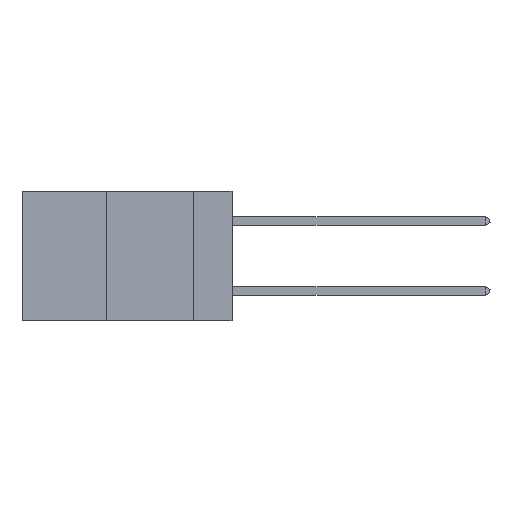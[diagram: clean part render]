
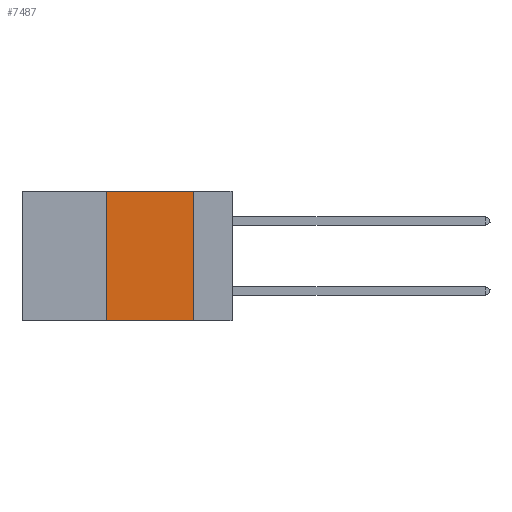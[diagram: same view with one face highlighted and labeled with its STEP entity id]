
A CAD part, left-side view. The second image highlights one B-rep face of the part: STEP entity #7487.
In plain terms, the highlighted planar face has unit normal (-1, 0, 0).
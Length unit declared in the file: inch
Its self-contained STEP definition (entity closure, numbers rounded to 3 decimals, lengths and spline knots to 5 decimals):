
#118 = VECTOR ( 'NONE', #20390, 39.37008 ) ;
#226 = ORIENTED_EDGE ( 'NONE', *, *, #33072, .F. ) ;
#620 = PLANE ( 'NONE',  #11487 ) ;
#1756 = LINE ( 'NONE', #30746, #118 ) ;
#3171 = VECTOR ( 'NONE', #6409, 39.37008 ) ;
#4182 = EDGE_CURVE ( 'NONE', #19419, #30702, #10071, .T. ) ;
#4533 = CARTESIAN_POINT ( 'NONE',  ( 0., 0.11, 0. ) ) ;
#4989 = CARTESIAN_POINT ( 'NONE',  ( 0., 0.6, -0.37 ) ) ;
#5253 = LINE ( 'NONE', #30614, #9282 ) ;
#5281 = CARTESIAN_POINT ( 'NONE',  ( 0., 0.36, -0.37 ) ) ;
#6409 = DIRECTION ( 'NONE',  ( 0., 0., 1. ) ) ;
#6517 = LINE ( 'NONE', #4989, #19477 ) ;
#6552 = CARTESIAN_POINT ( 'NONE',  ( 0., 0.11, -0.37 ) ) ;
#7487 = ADVANCED_FACE ( 'NONE', ( #15484 ), #620, .F. ) ;
#8469 = EDGE_CURVE ( 'NONE', #19419, #27528, #6517, .T. ) ;
#9282 = VECTOR ( 'NONE', #9524, 39.37008 ) ;
#9524 = DIRECTION ( 'NONE',  ( 0., 0., -1. ) ) ;
#9711 = VERTEX_POINT ( 'NONE', #4533 ) ;
#10071 = LINE ( 'NONE', #16402, #3171 ) ;
#11487 = AXIS2_PLACEMENT_3D ( 'NONE', #21248, #29193, #29083 ) ;
#11657 = CARTESIAN_POINT ( 'NONE',  ( 0., 0.36, 0. ) ) ;
#13347 = ORIENTED_EDGE ( 'NONE', *, *, #4182, .F. ) ;
#15484 = FACE_OUTER_BOUND ( 'NONE', #20965, .T. ) ;
#16402 = CARTESIAN_POINT ( 'NONE',  ( 0., 0.36, 0. ) ) ;
#18621 = EDGE_CURVE ( 'NONE', #9711, #27528, #5253, .T. ) ;
#19419 = VERTEX_POINT ( 'NONE', #5281 ) ;
#19477 = VECTOR ( 'NONE', #23463, 39.37008 ) ;
#20125 = ORIENTED_EDGE ( 'NONE', *, *, #18621, .F. ) ;
#20390 = DIRECTION ( 'NONE',  ( 0., -1., 0. ) ) ;
#20965 = EDGE_LOOP ( 'NONE', ( #20125, #226, #13347, #32925 ) ) ;
#21248 = CARTESIAN_POINT ( 'NONE',  ( 0., 0.6, 0. ) ) ;
#23463 = DIRECTION ( 'NONE',  ( 0., -1., 0. ) ) ;
#27528 = VERTEX_POINT ( 'NONE', #6552 ) ;
#29083 = DIRECTION ( 'NONE',  ( 0., 0., -1. ) ) ;
#29193 = DIRECTION ( 'NONE',  ( 1., 0., 0. ) ) ;
#30614 = CARTESIAN_POINT ( 'NONE',  ( 0., 0.11, 0. ) ) ;
#30702 = VERTEX_POINT ( 'NONE', #11657 ) ;
#30746 = CARTESIAN_POINT ( 'NONE',  ( 0., 0.6, 0. ) ) ;
#32925 = ORIENTED_EDGE ( 'NONE', *, *, #8469, .T. ) ;
#33072 = EDGE_CURVE ( 'NONE', #30702, #9711, #1756, .T. ) ;
